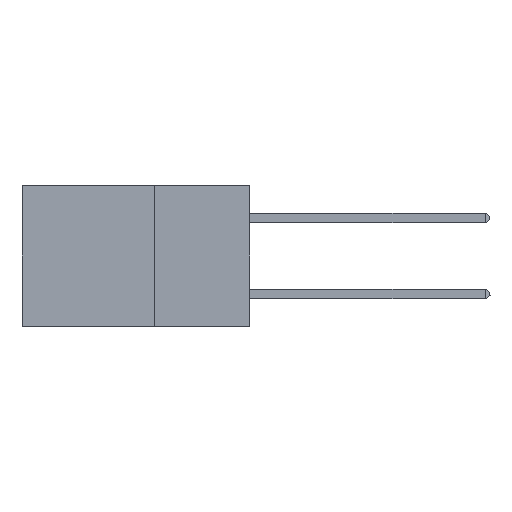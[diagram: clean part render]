
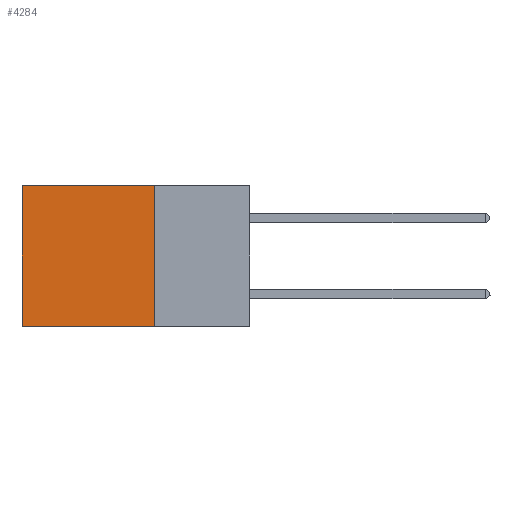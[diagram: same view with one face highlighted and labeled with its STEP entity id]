
A CAD part, left-side view. The second image highlights one B-rep face of the part: STEP entity #4284.
In plain terms, the highlighted planar face has unit normal (-1, 0, 0).
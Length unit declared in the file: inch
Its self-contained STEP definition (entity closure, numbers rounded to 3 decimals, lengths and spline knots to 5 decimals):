
#368 = CARTESIAN_POINT ( 'NONE',  ( 0.2875, 0.25, 0. ) ) ;
#1204 = LINE ( 'NONE', #3213, #13665 ) ;
#2925 = VERTEX_POINT ( 'NONE', #6505 ) ;
#3213 = CARTESIAN_POINT ( 'NONE',  ( 0.2875, 0.25, 0. ) ) ;
#3860 = DIRECTION ( 'NONE',  ( 0., 0., -1. ) ) ;
#4284 = ADVANCED_FACE ( 'NONE', ( #12589 ), #18302, .F. ) ;
#4456 = LINE ( 'NONE', #18382, #15202 ) ;
#4998 = LINE ( 'NONE', #14307, #7883 ) ;
#5403 = VERTEX_POINT ( 'NONE', #13920 ) ;
#6156 = ORIENTED_EDGE ( 'NONE', *, *, #15542, .F. ) ;
#6505 = CARTESIAN_POINT ( 'NONE',  ( 0.2875, 0.25, 0. ) ) ;
#7807 = DIRECTION ( 'NONE',  ( 0., 1., 0. ) ) ;
#7883 = VECTOR ( 'NONE', #15770, 39.37008 ) ;
#8343 = EDGE_LOOP ( 'NONE', ( #9967, #19274, #6156, #15499 ) ) ;
#9476 = DIRECTION ( 'NONE',  ( 0., 0., -1. ) ) ;
#9967 = ORIENTED_EDGE ( 'NONE', *, *, #18831, .T. ) ;
#11334 = VECTOR ( 'NONE', #3860, 39.37008 ) ;
#11587 = VERTEX_POINT ( 'NONE', #11833 ) ;
#11833 = CARTESIAN_POINT ( 'NONE',  ( 0.2875, 0.6, -0.37 ) ) ;
#12012 = EDGE_CURVE ( 'NONE', #17619, #11587, #4998, .T. ) ;
#12103 = DIRECTION ( 'NONE',  ( 0., 0., -1. ) ) ;
#12286 = LINE ( 'NONE', #19137, #11334 ) ;
#12589 = FACE_OUTER_BOUND ( 'NONE', #8343, .T. ) ;
#13665 = VECTOR ( 'NONE', #7807, 39.37008 ) ;
#13920 = CARTESIAN_POINT ( 'NONE',  ( 0.2875, 0.6, 0. ) ) ;
#14307 = CARTESIAN_POINT ( 'NONE',  ( 0.2875, 0.25, -0.37 ) ) ;
#14964 = AXIS2_PLACEMENT_3D ( 'NONE', #368, #15569, #9476 ) ;
#15202 = VECTOR ( 'NONE', #12103, 39.37008 ) ;
#15499 = ORIENTED_EDGE ( 'NONE', *, *, #16479, .T. ) ;
#15542 = EDGE_CURVE ( 'NONE', #2925, #17619, #12286, .T. ) ;
#15569 = DIRECTION ( 'NONE',  ( 1., 0., 0. ) ) ;
#15638 = CARTESIAN_POINT ( 'NONE',  ( 0.2875, 0.25, -0.37 ) ) ;
#15770 = DIRECTION ( 'NONE',  ( 0., 1., 0. ) ) ;
#16479 = EDGE_CURVE ( 'NONE', #2925, #5403, #1204, .T. ) ;
#17619 = VERTEX_POINT ( 'NONE', #15638 ) ;
#18302 = PLANE ( 'NONE',  #14964 ) ;
#18382 = CARTESIAN_POINT ( 'NONE',  ( 0.2875, 0.6, 0. ) ) ;
#18831 = EDGE_CURVE ( 'NONE', #5403, #11587, #4456, .T. ) ;
#19137 = CARTESIAN_POINT ( 'NONE',  ( 0.2875, 0.25, 0. ) ) ;
#19274 = ORIENTED_EDGE ( 'NONE', *, *, #12012, .F. ) ;
